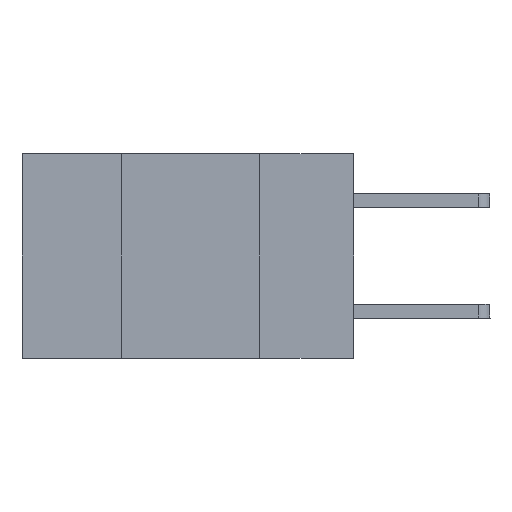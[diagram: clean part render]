
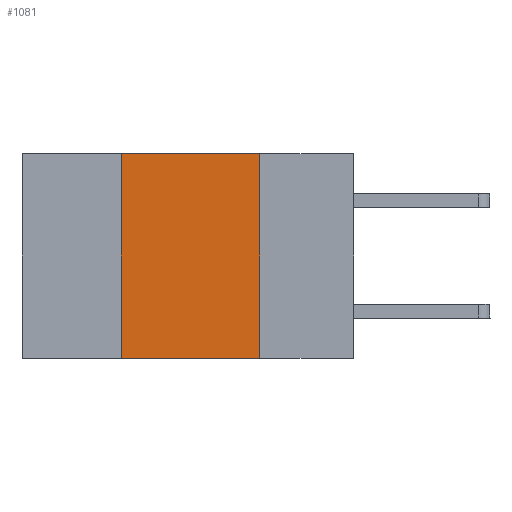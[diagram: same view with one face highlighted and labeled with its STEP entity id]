
A CAD part, left-side view. The second image highlights one B-rep face of the part: STEP entity #1081.
In plain terms, the highlighted planar face has unit normal (-1, 0, 0).
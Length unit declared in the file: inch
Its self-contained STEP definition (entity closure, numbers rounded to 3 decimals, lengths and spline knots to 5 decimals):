
#176 = CARTESIAN_POINT ( 'NONE',  ( 0., 0.42, -0.37 ) ) ;
#286 = LINE ( 'NONE', #550, #846 ) ;
#353 = CARTESIAN_POINT ( 'NONE',  ( 0., 0.17, 0. ) ) ;
#381 = CARTESIAN_POINT ( 'NONE',  ( 0., 0.6, 0. ) ) ;
#550 = CARTESIAN_POINT ( 'NONE',  ( 0., 0.17, 0. ) ) ;
#846 = VECTOR ( 'NONE', #2221, 39.37008 ) ;
#1081 = ADVANCED_FACE ( 'NONE', ( #6031 ), #10735, .F. ) ;
#1641 = VERTEX_POINT ( 'NONE', #8321 ) ;
#1909 = DIRECTION ( 'NONE',  ( 0., -1., 0. ) ) ;
#2164 = DIRECTION ( 'NONE',  ( 0., 0., -1. ) ) ;
#2221 = DIRECTION ( 'NONE',  ( 0., 0., -1. ) ) ;
#2342 = VECTOR ( 'NONE', #3386, 39.37008 ) ;
#2666 = EDGE_CURVE ( 'NONE', #1641, #10609, #7774, .T. ) ;
#2749 = CARTESIAN_POINT ( 'NONE',  ( 0., 0.42, 0. ) ) ;
#2938 = EDGE_LOOP ( 'NONE', ( #6144, #9174, #9372, #7320 ) ) ;
#3014 = VECTOR ( 'NONE', #1909, 39.37008 ) ;
#3038 = AXIS2_PLACEMENT_3D ( 'NONE', #381, #3848, #2164 ) ;
#3386 = DIRECTION ( 'NONE',  ( 0., -1., 0. ) ) ;
#3651 = LINE ( 'NONE', #9840, #3014 ) ;
#3848 = DIRECTION ( 'NONE',  ( 1., 0., 0. ) ) ;
#5106 = LINE ( 'NONE', #2749, #10549 ) ;
#5419 = EDGE_CURVE ( 'NONE', #9896, #5951, #3651, .T. ) ;
#5951 = VERTEX_POINT ( 'NONE', #6692 ) ;
#6031 = FACE_OUTER_BOUND ( 'NONE', #2938, .T. ) ;
#6144 = ORIENTED_EDGE ( 'NONE', *, *, #8974, .F. ) ;
#6692 = CARTESIAN_POINT ( 'NONE',  ( 0., 0.17, -0.37 ) ) ;
#6949 = DIRECTION ( 'NONE',  ( 0., 0., 1. ) ) ;
#7320 = ORIENTED_EDGE ( 'NONE', *, *, #5419, .T. ) ;
#7359 = EDGE_CURVE ( 'NONE', #9896, #1641, #5106, .T. ) ;
#7774 = LINE ( 'NONE', #11249, #2342 ) ;
#8321 = CARTESIAN_POINT ( 'NONE',  ( 0., 0.42, 0. ) ) ;
#8974 = EDGE_CURVE ( 'NONE', #10609, #5951, #286, .T. ) ;
#9174 = ORIENTED_EDGE ( 'NONE', *, *, #2666, .F. ) ;
#9372 = ORIENTED_EDGE ( 'NONE', *, *, #7359, .F. ) ;
#9840 = CARTESIAN_POINT ( 'NONE',  ( 0., 0.6, -0.37 ) ) ;
#9896 = VERTEX_POINT ( 'NONE', #176 ) ;
#10549 = VECTOR ( 'NONE', #6949, 39.37008 ) ;
#10609 = VERTEX_POINT ( 'NONE', #353 ) ;
#10735 = PLANE ( 'NONE',  #3038 ) ;
#11249 = CARTESIAN_POINT ( 'NONE',  ( 0., 0.6, 0. ) ) ;
